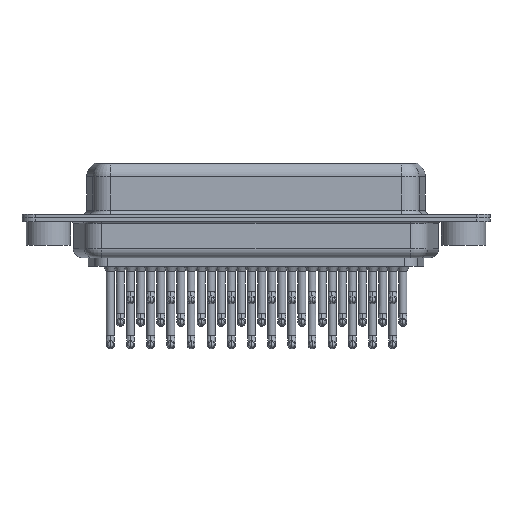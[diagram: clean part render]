
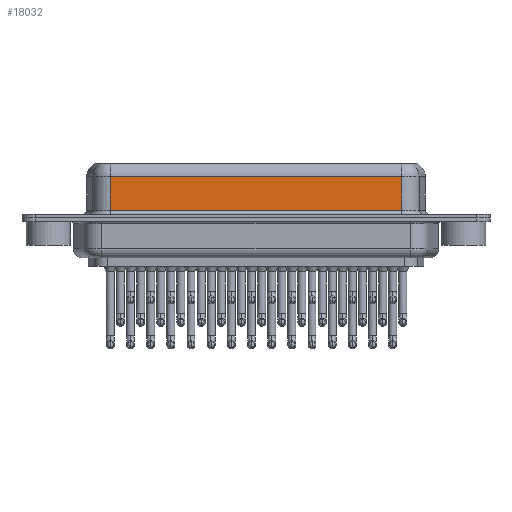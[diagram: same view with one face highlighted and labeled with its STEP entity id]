
A CAD part, front view. The second image highlights one B-rep face of the part: STEP entity #18032.
In plain terms, the highlighted planar face has unit normal (0, -1, 0).
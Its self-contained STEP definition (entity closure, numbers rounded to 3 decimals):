
#119 = CARTESIAN_POINT ( 'NONE',  ( 7.013, -3.95, 4.65 ) ) ;
#2001 = ORIENTED_EDGE ( 'NONE', *, *, #13788, .T. ) ;
#2024 = CARTESIAN_POINT ( 'NONE',  ( 40.037, -3.95, 0.9 ) ) ;
#2399 = PLANE ( 'NONE',  #10144 ) ;
#3073 = ORIENTED_EDGE ( 'NONE', *, *, #15056, .T. ) ;
#4137 = EDGE_LOOP ( 'NONE', ( #7138, #2001, #3073, #29832 ) ) ;
#4858 = DIRECTION ( 'NONE',  ( 0., 1., 0. ) ) ;
#5680 = DIRECTION ( 'NONE',  ( -1., 0., 0. ) ) ;
#6733 = DIRECTION ( 'NONE',  ( 1., 0., 0. ) ) ;
#6735 = VECTOR ( 'NONE', #6733, 1000. ) ;
#7138 = ORIENTED_EDGE ( 'NONE', *, *, #28716, .F. ) ;
#7590 = LINE ( 'NONE', #9548, #18845 ) ;
#8348 = EDGE_CURVE ( 'NONE', #10506, #17080, #20251, .T. ) ;
#9220 = DIRECTION ( 'NONE',  ( 0., 0., -1. ) ) ;
#9548 = CARTESIAN_POINT ( 'NONE',  ( 40.037, -3.95, 6.4 ) ) ;
#10144 = AXIS2_PLACEMENT_3D ( 'NONE', #19142, #4858, #21581 ) ;
#10506 = VERTEX_POINT ( 'NONE', #29177 ) ;
#13214 = FACE_OUTER_BOUND ( 'NONE', #4137, .T. ) ;
#13788 = EDGE_CURVE ( 'NONE', #17202, #26713, #15113, .T. ) ;
#15056 = EDGE_CURVE ( 'NONE', #26713, #10506, #21815, .T. ) ;
#15113 = LINE ( 'NONE', #24823, #26345 ) ;
#15408 = VECTOR ( 'NONE', #9220, 1000. ) ;
#17080 = VERTEX_POINT ( 'NONE', #21937 ) ;
#17202 = VERTEX_POINT ( 'NONE', #22351 ) ;
#18032 = ADVANCED_FACE ( 'NONE', ( #13214 ), #2399, .F. ) ;
#18845 = VECTOR ( 'NONE', #28748, 1000. ) ;
#19142 = CARTESIAN_POINT ( 'NONE',  ( 40.037, -3.95, 6.4 ) ) ;
#20251 = LINE ( 'NONE', #2024, #6735 ) ;
#21581 = DIRECTION ( 'NONE',  ( 0., 0., 1. ) ) ;
#21815 = LINE ( 'NONE', #26007, #15408 ) ;
#21937 = CARTESIAN_POINT ( 'NONE',  ( 40.037, -3.95, 0.9 ) ) ;
#22351 = CARTESIAN_POINT ( 'NONE',  ( 40.037, -3.95, 4.65 ) ) ;
#24823 = CARTESIAN_POINT ( 'NONE',  ( 40.037, -3.95, 4.65 ) ) ;
#26007 = CARTESIAN_POINT ( 'NONE',  ( 7.013, -3.95, 6.4 ) ) ;
#26345 = VECTOR ( 'NONE', #5680, 1000. ) ;
#26713 = VERTEX_POINT ( 'NONE', #119 ) ;
#28716 = EDGE_CURVE ( 'NONE', #17202, #17080, #7590, .T. ) ;
#28748 = DIRECTION ( 'NONE',  ( 0., 0., -1. ) ) ;
#29177 = CARTESIAN_POINT ( 'NONE',  ( 7.013, -3.95, 0.9 ) ) ;
#29832 = ORIENTED_EDGE ( 'NONE', *, *, #8348, .T. ) ;
